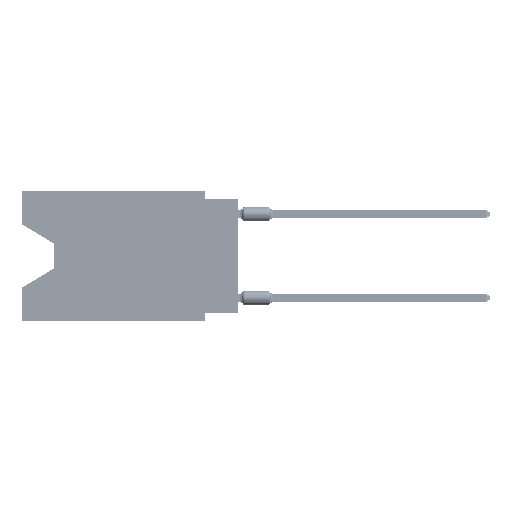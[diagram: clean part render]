
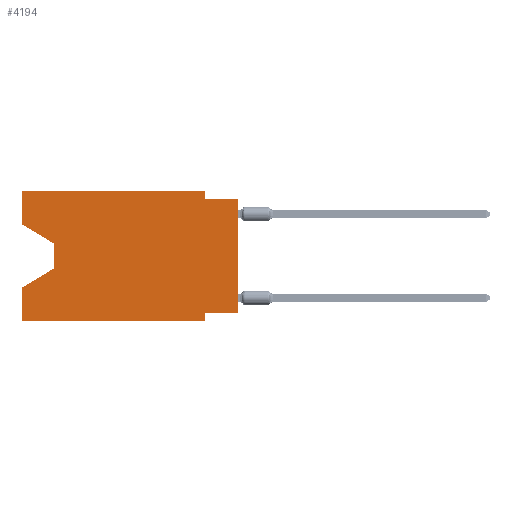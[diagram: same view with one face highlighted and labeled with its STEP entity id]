
A CAD part, left-side view. The second image highlights one B-rep face of the part: STEP entity #4194.
In plain terms, the highlighted planar face has unit normal (-1, 0, 0).
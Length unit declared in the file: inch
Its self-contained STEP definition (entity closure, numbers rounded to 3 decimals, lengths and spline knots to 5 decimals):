
#488 = LINE ( 'NONE', #60113, #50501 ) ;
#698 = EDGE_CURVE ( 'NONE', #73913, #78263, #70995, .T. ) ;
#2477 = LINE ( 'NONE', #62523, #75879 ) ;
#2803 = DIRECTION ( 'NONE',  ( 1., 0., 0. ) ) ;
#4075 = CARTESIAN_POINT ( 'NONE',  ( 0., 0.645, -0.39 ) ) ;
#4194 = ADVANCED_FACE ( 'NONE', ( #29737 ), #49593, .F. ) ;
#4595 = DIRECTION ( 'NONE',  ( 0., 1., 0. ) ) ;
#5168 = VECTOR ( 'NONE', #24438, 39.37008 ) ;
#5329 = LINE ( 'NONE', #18158, #79544 ) ;
#5443 = CARTESIAN_POINT ( 'NONE',  ( 0., 0.645, -0.10025 ) ) ;
#8737 = VECTOR ( 'NONE', #55017, 39.37008 ) ;
#9439 = CARTESIAN_POINT ( 'NONE',  ( 0., 0.645, 0. ) ) ;
#11332 = CARTESIAN_POINT ( 'NONE',  ( 0., 0.55, -0.232 ) ) ;
#12347 = EDGE_CURVE ( 'NONE', #36954, #44381, #48293, .T. ) ;
#14422 = CARTESIAN_POINT ( 'NONE',  ( 0., 0., -0.025 ) ) ;
#14560 = CARTESIAN_POINT ( 'NONE',  ( 0., 0., 0. ) ) ;
#15280 = DIRECTION ( 'NONE',  ( 0., 0., 1. ) ) ;
#15841 = ORIENTED_EDGE ( 'NONE', *, *, #48461, .T. ) ;
#16025 = DIRECTION ( 'NONE',  ( 0., -1., 0. ) ) ;
#16775 = CARTESIAN_POINT ( 'NONE',  ( 0., 0.1, -0.365 ) ) ;
#16831 = EDGE_CURVE ( 'NONE', #38713, #17680, #38605, .T. ) ;
#17680 = VERTEX_POINT ( 'NONE', #16775 ) ;
#18158 = CARTESIAN_POINT ( 'NONE',  ( 0., 0.645, 0. ) ) ;
#18285 = VECTOR ( 'NONE', #71429, 39.37008 ) ;
#18710 = VECTOR ( 'NONE', #50925, 39.37008 ) ;
#20729 = CARTESIAN_POINT ( 'NONE',  ( 0., 0.1, -0.39 ) ) ;
#24416 = VERTEX_POINT ( 'NONE', #77933 ) ;
#24438 = DIRECTION ( 'NONE',  ( 0., 0., 1. ) ) ;
#25036 = ORIENTED_EDGE ( 'NONE', *, *, #698, .F. ) ;
#25315 = LINE ( 'NONE', #5443, #18710 ) ;
#26810 = VERTEX_POINT ( 'NONE', #76331 ) ;
#26969 = VECTOR ( 'NONE', #4595, 39.37008 ) ;
#28252 = DIRECTION ( 'NONE',  ( 0., 0., 1. ) ) ;
#28670 = ORIENTED_EDGE ( 'NONE', *, *, #85103, .F. ) ;
#29737 = FACE_OUTER_BOUND ( 'NONE', #54498, .T. ) ;
#30897 = EDGE_CURVE ( 'NONE', #24416, #36940, #488, .T. ) ;
#33564 = CARTESIAN_POINT ( 'NONE',  ( 0., 0.1, -0.025 ) ) ;
#33663 = CARTESIAN_POINT ( 'NONE',  ( 0., 0.645, -0.39 ) ) ;
#36940 = VERTEX_POINT ( 'NONE', #53938 ) ;
#36954 = VERTEX_POINT ( 'NONE', #33663 ) ;
#37197 = LINE ( 'NONE', #4075, #53383 ) ;
#37846 = LINE ( 'NONE', #11332, #74374 ) ;
#38605 = LINE ( 'NONE', #84944, #26969 ) ;
#38713 = VERTEX_POINT ( 'NONE', #48976 ) ;
#39752 = DIRECTION ( 'NONE',  ( 0., -1., 0. ) ) ;
#43274 = ORIENTED_EDGE ( 'NONE', *, *, #79255, .F. ) ;
#43914 = EDGE_CURVE ( 'NONE', #17680, #71088, #77236, .T. ) ;
#44381 = VERTEX_POINT ( 'NONE', #70939 ) ;
#44500 = CARTESIAN_POINT ( 'NONE',  ( 0., 0.1, 0. ) ) ;
#47139 = ORIENTED_EDGE ( 'NONE', *, *, #43914, .F. ) ;
#48217 = VERTEX_POINT ( 'NONE', #54654 ) ;
#48261 = AXIS2_PLACEMENT_3D ( 'NONE', #9439, #2803, #83593 ) ;
#48293 = LINE ( 'NONE', #75234, #5168 ) ;
#48461 = EDGE_CURVE ( 'NONE', #36940, #44381, #37846, .T. ) ;
#48976 = CARTESIAN_POINT ( 'NONE',  ( 0., 0., -0.365 ) ) ;
#49472 = CARTESIAN_POINT ( 'NONE',  ( 0., 0.645, 0. ) ) ;
#49593 = PLANE ( 'NONE',  #48261 ) ;
#50501 = VECTOR ( 'NONE', #87032, 39.37008 ) ;
#50925 = DIRECTION ( 'NONE',  ( 0., -0.855, -0.519 ) ) ;
#51077 = DIRECTION ( 'NONE',  ( 0., 0.855, -0.519 ) ) ;
#53383 = VECTOR ( 'NONE', #16025, 39.37008 ) ;
#53792 = ORIENTED_EDGE ( 'NONE', *, *, #12347, .F. ) ;
#53938 = CARTESIAN_POINT ( 'NONE',  ( 0., 0.55, -0.232 ) ) ;
#54498 = EDGE_LOOP ( 'NONE', ( #86349, #83975, #15841, #53792, #66811, #47139, #83767, #76739, #28670, #25036, #68822, #43274 ) ) ;
#54654 = CARTESIAN_POINT ( 'NONE',  ( 0., 0., -0.025 ) ) ;
#55017 = DIRECTION ( 'NONE',  ( 0., -1., 0. ) ) ;
#56043 = CARTESIAN_POINT ( 'NONE',  ( 0., 0.1, -0.39 ) ) ;
#57744 = EDGE_CURVE ( 'NONE', #36954, #71088, #37197, .T. ) ;
#60113 = CARTESIAN_POINT ( 'NONE',  ( 0., 0.55, -0.158 ) ) ;
#61366 = LINE ( 'NONE', #14560, #80857 ) ;
#62523 = CARTESIAN_POINT ( 'NONE',  ( 0., 0.645, 0. ) ) ;
#63448 = CARTESIAN_POINT ( 'NONE',  ( 0., 0.1, 0. ) ) ;
#65311 = EDGE_CURVE ( 'NONE', #38713, #48217, #61366, .T. ) ;
#66811 = ORIENTED_EDGE ( 'NONE', *, *, #57744, .T. ) ;
#67911 = EDGE_CURVE ( 'NONE', #74985, #73913, #5329, .T. ) ;
#68822 = ORIENTED_EDGE ( 'NONE', *, *, #67911, .F. ) ;
#70939 = CARTESIAN_POINT ( 'NONE',  ( 0., 0.645, -0.28975 ) ) ;
#70995 = LINE ( 'NONE', #44500, #18285 ) ;
#71088 = VERTEX_POINT ( 'NONE', #20729 ) ;
#71429 = DIRECTION ( 'NONE',  ( 0., 0., -1. ) ) ;
#73913 = VERTEX_POINT ( 'NONE', #63448 ) ;
#74374 = VECTOR ( 'NONE', #51077, 39.37008 ) ;
#74985 = VERTEX_POINT ( 'NONE', #49472 ) ;
#75234 = CARTESIAN_POINT ( 'NONE',  ( 0., 0.645, 0. ) ) ;
#75879 = VECTOR ( 'NONE', #15280, 39.37008 ) ;
#76331 = CARTESIAN_POINT ( 'NONE',  ( 0., 0.645, -0.10025 ) ) ;
#76739 = ORIENTED_EDGE ( 'NONE', *, *, #65311, .T. ) ;
#77236 = LINE ( 'NONE', #56043, #86512 ) ;
#77933 = CARTESIAN_POINT ( 'NONE',  ( 0., 0.55, -0.158 ) ) ;
#78263 = VERTEX_POINT ( 'NONE', #33564 ) ;
#79255 = EDGE_CURVE ( 'NONE', #26810, #74985, #2477, .T. ) ;
#79544 = VECTOR ( 'NONE', #39752, 39.37008 ) ;
#80857 = VECTOR ( 'NONE', #28252, 39.37008 ) ;
#81095 = LINE ( 'NONE', #14422, #8737 ) ;
#83593 = DIRECTION ( 'NONE',  ( 0., 0., -1. ) ) ;
#83767 = ORIENTED_EDGE ( 'NONE', *, *, #16831, .F. ) ;
#83848 = DIRECTION ( 'NONE',  ( 0., 0., -1. ) ) ;
#83975 = ORIENTED_EDGE ( 'NONE', *, *, #30897, .T. ) ;
#84944 = CARTESIAN_POINT ( 'NONE',  ( 0., 0., -0.365 ) ) ;
#85103 = EDGE_CURVE ( 'NONE', #78263, #48217, #81095, .T. ) ;
#85803 = EDGE_CURVE ( 'NONE', #26810, #24416, #25315, .T. ) ;
#86349 = ORIENTED_EDGE ( 'NONE', *, *, #85803, .T. ) ;
#86512 = VECTOR ( 'NONE', #83848, 39.37008 ) ;
#87032 = DIRECTION ( 'NONE',  ( 0., 0., -1. ) ) ;
